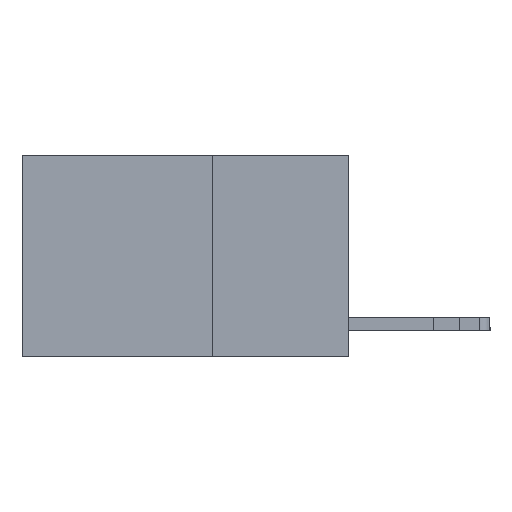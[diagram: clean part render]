
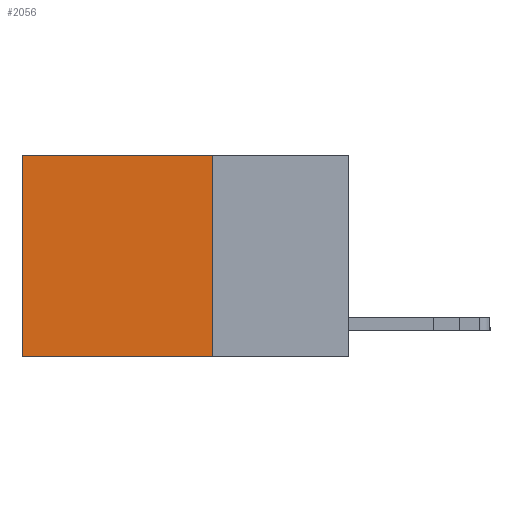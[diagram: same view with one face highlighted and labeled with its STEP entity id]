
A CAD part, left-side view. The second image highlights one B-rep face of the part: STEP entity #2056.
In plain terms, the highlighted planar face has unit normal (-1, 0, 0).
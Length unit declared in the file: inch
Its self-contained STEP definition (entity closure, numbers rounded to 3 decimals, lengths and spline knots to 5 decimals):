
#1216 = ORIENTED_EDGE ( 'NONE', *, *, #9167, .T. ) ;
#1517 = EDGE_CURVE ( 'NONE', #10648, #17148, #3744, .T. ) ;
#2056 = ADVANCED_FACE ( 'NONE', ( #16642 ), #2317, .F. ) ;
#2209 = CARTESIAN_POINT ( 'NONE',  ( 0.2625, 0.25, 0. ) ) ;
#2317 = PLANE ( 'NONE',  #11413 ) ;
#3140 = LINE ( 'NONE', #4999, #15482 ) ;
#3744 = LINE ( 'NONE', #13354, #17060 ) ;
#4999 = CARTESIAN_POINT ( 'NONE',  ( 0.2625, 0.25, 0. ) ) ;
#5867 = DIRECTION ( 'NONE',  ( 1., 0., 0. ) ) ;
#6084 = CARTESIAN_POINT ( 'NONE',  ( 0.2625, 0.6, -0.37 ) ) ;
#6101 = DIRECTION ( 'NONE',  ( 0., 0., -1. ) ) ;
#6447 = EDGE_CURVE ( 'NONE', #14436, #10648, #17180, .T. ) ;
#7765 = CARTESIAN_POINT ( 'NONE',  ( 0.2625, 0.25, 0. ) ) ;
#7838 = DIRECTION ( 'NONE',  ( 0., 0., -1. ) ) ;
#8751 = CARTESIAN_POINT ( 'NONE',  ( 0.2625, 0.25, -0.37 ) ) ;
#9167 = EDGE_CURVE ( 'NONE', #15167, #17148, #19105, .T. ) ;
#9242 = DIRECTION ( 'NONE',  ( 0., 0., -1. ) ) ;
#9885 = CARTESIAN_POINT ( 'NONE',  ( 0.2625, 0.6, 0. ) ) ;
#10648 = VERTEX_POINT ( 'NONE', #8751 ) ;
#11413 = AXIS2_PLACEMENT_3D ( 'NONE', #15075, #5867, #7838 ) ;
#11661 = EDGE_CURVE ( 'NONE', #14436, #15167, #3140, .T. ) ;
#12561 = VECTOR ( 'NONE', #6101, 39.37008 ) ;
#13354 = CARTESIAN_POINT ( 'NONE',  ( 0.2625, 0.25, -0.37 ) ) ;
#13711 = ORIENTED_EDGE ( 'NONE', *, *, #6447, .F. ) ;
#14436 = VERTEX_POINT ( 'NONE', #2209 ) ;
#15075 = CARTESIAN_POINT ( 'NONE',  ( 0.2625, 0.25, 0. ) ) ;
#15167 = VERTEX_POINT ( 'NONE', #9885 ) ;
#15482 = VECTOR ( 'NONE', #20492, 39.37008 ) ;
#15603 = CARTESIAN_POINT ( 'NONE',  ( 0.2625, 0.6, 0. ) ) ;
#16642 = FACE_OUTER_BOUND ( 'NONE', #19219, .T. ) ;
#16936 = ORIENTED_EDGE ( 'NONE', *, *, #11661, .T. ) ;
#17060 = VECTOR ( 'NONE', #18659, 39.37008 ) ;
#17148 = VERTEX_POINT ( 'NONE', #6084 ) ;
#17180 = LINE ( 'NONE', #7765, #12561 ) ;
#17760 = VECTOR ( 'NONE', #9242, 39.37008 ) ;
#18659 = DIRECTION ( 'NONE',  ( 0., 1., 0. ) ) ;
#19105 = LINE ( 'NONE', #15603, #17760 ) ;
#19219 = EDGE_LOOP ( 'NONE', ( #1216, #19920, #13711, #16936 ) ) ;
#19920 = ORIENTED_EDGE ( 'NONE', *, *, #1517, .F. ) ;
#20492 = DIRECTION ( 'NONE',  ( 0., 1., 0. ) ) ;
